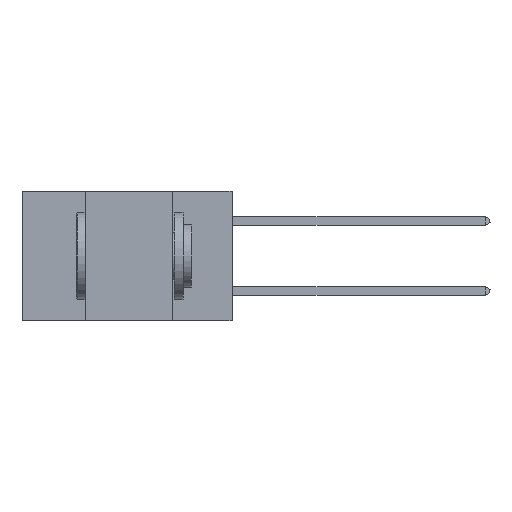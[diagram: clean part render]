
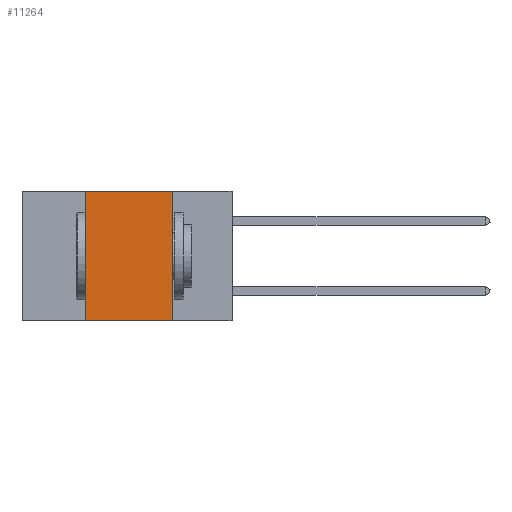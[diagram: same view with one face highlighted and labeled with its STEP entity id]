
A CAD part, left-side view. The second image highlights one B-rep face of the part: STEP entity #11264.
In plain terms, the highlighted planar face has unit normal (-1, 0, 0).
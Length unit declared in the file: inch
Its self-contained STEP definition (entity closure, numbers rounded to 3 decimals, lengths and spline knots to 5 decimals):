
#2646 = CARTESIAN_POINT ( 'NONE',  ( 0., 0.42, 0. ) ) ;
#2655 = DIRECTION ( 'NONE',  ( 0., -1., 0. ) ) ;
#4180 = DIRECTION ( 'NONE',  ( 0., -1., 0. ) ) ;
#4536 = VECTOR ( 'NONE', #28528, 39.37008 ) ;
#5473 = VECTOR ( 'NONE', #2655, 39.37008 ) ;
#6798 = EDGE_CURVE ( 'NONE', #11848, #33727, #25844, .T. ) ;
#7350 = PLANE ( 'NONE',  #19680 ) ;
#9099 = ORIENTED_EDGE ( 'NONE', *, *, #6798, .F. ) ;
#9707 = CARTESIAN_POINT ( 'NONE',  ( 0., 0.17, 0. ) ) ;
#11082 = ORIENTED_EDGE ( 'NONE', *, *, #19198, .F. ) ;
#11258 = FACE_OUTER_BOUND ( 'NONE', #33013, .T. ) ;
#11264 = ADVANCED_FACE ( 'NONE', ( #11258 ), #7350, .F. ) ;
#11848 = VERTEX_POINT ( 'NONE', #9707 ) ;
#12238 = CARTESIAN_POINT ( 'NONE',  ( 0., 0.17, -0.37 ) ) ;
#16126 = LINE ( 'NONE', #25151, #4536 ) ;
#17286 = EDGE_CURVE ( 'NONE', #27320, #33727, #34279, .T. ) ;
#18839 = DIRECTION ( 'NONE',  ( 1., 0., 0. ) ) ;
#18903 = VECTOR ( 'NONE', #37278, 39.37008 ) ;
#18974 = EDGE_CURVE ( 'NONE', #27320, #34225, #16126, .T. ) ;
#19173 = CARTESIAN_POINT ( 'NONE',  ( 0., 0.6, -0.37 ) ) ;
#19198 = EDGE_CURVE ( 'NONE', #34225, #11848, #21164, .T. ) ;
#19680 = AXIS2_PLACEMENT_3D ( 'NONE', #36650, #18839, #28031 ) ;
#20024 = ORIENTED_EDGE ( 'NONE', *, *, #17286, .T. ) ;
#20546 = ORIENTED_EDGE ( 'NONE', *, *, #18974, .F. ) ;
#21164 = LINE ( 'NONE', #36450, #5473 ) ;
#25151 = CARTESIAN_POINT ( 'NONE',  ( 0., 0.42, 0. ) ) ;
#25844 = LINE ( 'NONE', #30023, #18903 ) ;
#26711 = CARTESIAN_POINT ( 'NONE',  ( 0., 0.42, -0.37 ) ) ;
#27320 = VERTEX_POINT ( 'NONE', #26711 ) ;
#28031 = DIRECTION ( 'NONE',  ( 0., 0., -1. ) ) ;
#28528 = DIRECTION ( 'NONE',  ( 0., 0., 1. ) ) ;
#30023 = CARTESIAN_POINT ( 'NONE',  ( 0., 0.17, 0. ) ) ;
#33013 = EDGE_LOOP ( 'NONE', ( #9099, #11082, #20546, #20024 ) ) ;
#33727 = VERTEX_POINT ( 'NONE', #12238 ) ;
#34225 = VERTEX_POINT ( 'NONE', #2646 ) ;
#34279 = LINE ( 'NONE', #19173, #37048 ) ;
#36450 = CARTESIAN_POINT ( 'NONE',  ( 0., 0.6, 0. ) ) ;
#36650 = CARTESIAN_POINT ( 'NONE',  ( 0., 0.6, 0. ) ) ;
#37048 = VECTOR ( 'NONE', #4180, 39.37008 ) ;
#37278 = DIRECTION ( 'NONE',  ( 0., 0., -1. ) ) ;
